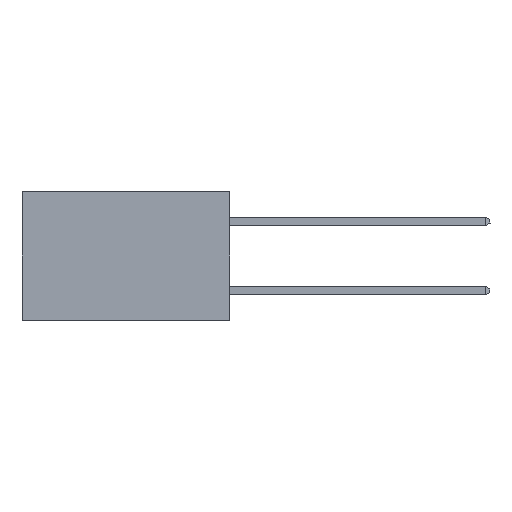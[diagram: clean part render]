
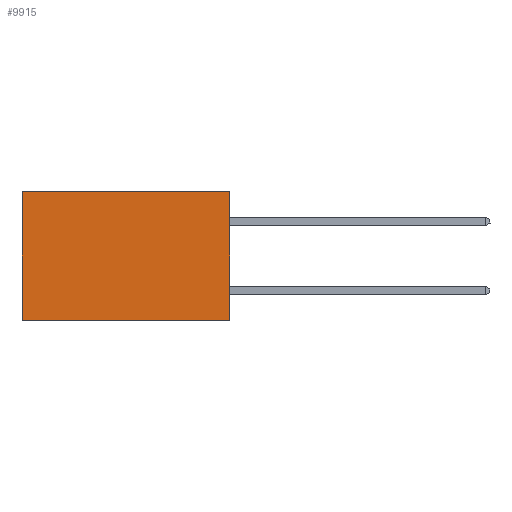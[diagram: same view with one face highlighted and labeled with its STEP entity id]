
A CAD part, left-side view. The second image highlights one B-rep face of the part: STEP entity #9915.
In plain terms, the highlighted planar face has unit normal (-1, 0, 0).
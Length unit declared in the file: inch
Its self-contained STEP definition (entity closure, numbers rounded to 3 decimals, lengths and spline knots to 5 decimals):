
#759 = LINE ( 'NONE', #22692, #22971 ) ;
#1361 = VERTEX_POINT ( 'NONE', #1387 ) ;
#1387 = CARTESIAN_POINT ( 'NONE',  ( 0.298, 0., 0. ) ) ;
#2397 = ORIENTED_EDGE ( 'NONE', *, *, #13840, .T. ) ;
#2914 = ORIENTED_EDGE ( 'NONE', *, *, #19686, .F. ) ;
#6714 = EDGE_LOOP ( 'NONE', ( #2397, #9770, #2914, #9969 ) ) ;
#9770 = ORIENTED_EDGE ( 'NONE', *, *, #28817, .F. ) ;
#9906 = LINE ( 'NONE', #25012, #13387 ) ;
#9915 = ADVANCED_FACE ( 'NONE', ( #24893 ), #17322, .F. ) ;
#9922 = CARTESIAN_POINT ( 'NONE',  ( 0.298, 0., 0. ) ) ;
#9969 = ORIENTED_EDGE ( 'NONE', *, *, #14716, .T. ) ;
#10599 = DIRECTION ( 'NONE',  ( 0., 0., -1. ) ) ;
#13387 = VECTOR ( 'NONE', #14965, 39.37008 ) ;
#13840 = EDGE_CURVE ( 'NONE', #14696, #15016, #759, .T. ) ;
#13971 = VECTOR ( 'NONE', #27031, 39.37008 ) ;
#14259 = VERTEX_POINT ( 'NONE', #32201 ) ;
#14696 = VERTEX_POINT ( 'NONE', #31852 ) ;
#14716 = EDGE_CURVE ( 'NONE', #1361, #14696, #20946, .T. ) ;
#14965 = DIRECTION ( 'NONE',  ( 0., 1., 0. ) ) ;
#15016 = VERTEX_POINT ( 'NONE', #16271 ) ;
#16271 = CARTESIAN_POINT ( 'NONE',  ( 0.298, 0.6, -0.37 ) ) ;
#17322 = PLANE ( 'NONE',  #28732 ) ;
#18668 = LINE ( 'NONE', #24481, #13971 ) ;
#19686 = EDGE_CURVE ( 'NONE', #1361, #14259, #18668, .T. ) ;
#20946 = LINE ( 'NONE', #29235, #27257 ) ;
#21787 = DIRECTION ( 'NONE',  ( 0., 1., 0. ) ) ;
#22209 = DIRECTION ( 'NONE',  ( 1., 0., 0. ) ) ;
#22692 = CARTESIAN_POINT ( 'NONE',  ( 0.298, 0.6, 0. ) ) ;
#22971 = VECTOR ( 'NONE', #10599, 39.37008 ) ;
#24481 = CARTESIAN_POINT ( 'NONE',  ( 0.298, 0., 0. ) ) ;
#24893 = FACE_OUTER_BOUND ( 'NONE', #6714, .T. ) ;
#25012 = CARTESIAN_POINT ( 'NONE',  ( 0.298, 0., -0.37 ) ) ;
#27031 = DIRECTION ( 'NONE',  ( 0., 0., -1. ) ) ;
#27257 = VECTOR ( 'NONE', #21787, 39.37008 ) ;
#28732 = AXIS2_PLACEMENT_3D ( 'NONE', #9922, #22209, #32291 ) ;
#28817 = EDGE_CURVE ( 'NONE', #14259, #15016, #9906, .T. ) ;
#29235 = CARTESIAN_POINT ( 'NONE',  ( 0.298, 0., 0. ) ) ;
#31852 = CARTESIAN_POINT ( 'NONE',  ( 0.298, 0.6, 0. ) ) ;
#32201 = CARTESIAN_POINT ( 'NONE',  ( 0.298, 0., -0.37 ) ) ;
#32291 = DIRECTION ( 'NONE',  ( 0., 0., -1. ) ) ;
